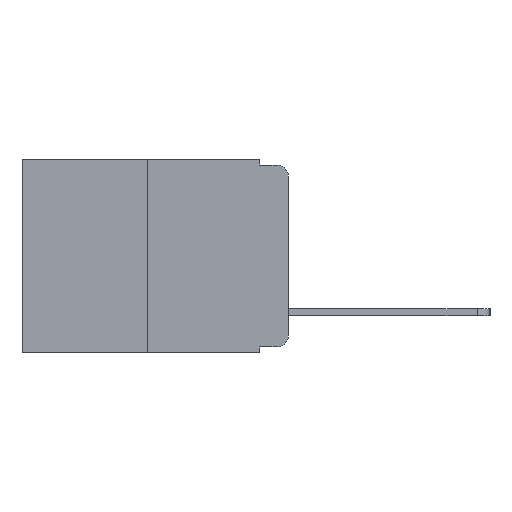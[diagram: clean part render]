
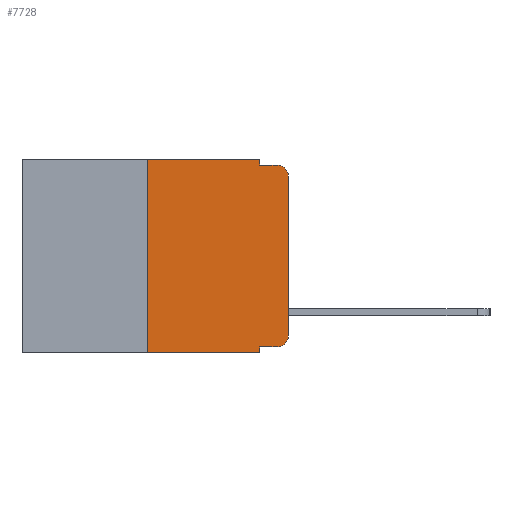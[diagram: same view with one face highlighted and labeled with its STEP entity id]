
A CAD part, left-side view. The second image highlights one B-rep face of the part: STEP entity #7728.
In plain terms, the highlighted planar face has unit normal (-1, 0, 0).
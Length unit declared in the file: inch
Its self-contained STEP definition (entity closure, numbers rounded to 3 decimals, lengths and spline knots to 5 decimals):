
#98 = DIRECTION ( 'NONE',  ( 0., -1., 0. ) ) ;
#183 = DIRECTION ( 'NONE',  ( 0., 0., -1. ) ) ;
#267 = ORIENTED_EDGE ( 'NONE', *, *, #5703, .T. ) ;
#307 = EDGE_CURVE ( 'NONE', #10371, #6859, #8863, .T. ) ;
#336 = CARTESIAN_POINT ( 'NONE',  ( 0., 0.473, 0. ) ) ;
#429 = LINE ( 'NONE', #5321, #7722 ) ;
#597 = ORIENTED_EDGE ( 'NONE', *, *, #5041, .T. ) ;
#945 = ORIENTED_EDGE ( 'NONE', *, *, #9875, .T. ) ;
#980 = ORIENTED_EDGE ( 'NONE', *, *, #4380, .F. ) ;
#998 = EDGE_CURVE ( 'NONE', #8926, #10371, #9156, .T. ) ;
#1080 = ORIENTED_EDGE ( 'NONE', *, *, #10041, .F. ) ;
#1398 = DIRECTION ( 'NONE',  ( 0., 0., -1. ) ) ;
#1710 = VECTOR ( 'NONE', #2047, 39.37008 ) ;
#1717 = EDGE_CURVE ( 'NONE', #8926, #1913, #6470, .T. ) ;
#1743 = ORIENTED_EDGE ( 'NONE', *, *, #307, .T. ) ;
#1839 = LINE ( 'NONE', #11655, #6770 ) ;
#1913 = VERTEX_POINT ( 'NONE', #4259 ) ;
#2047 = DIRECTION ( 'NONE',  ( 0., -1., 0. ) ) ;
#2114 = ORIENTED_EDGE ( 'NONE', *, *, #2402, .F. ) ;
#2126 = ORIENTED_EDGE ( 'NONE', *, *, #998, .T. ) ;
#2197 = CARTESIAN_POINT ( 'NONE',  ( 0., 0.473, 0. ) ) ;
#2402 = EDGE_CURVE ( 'NONE', #5201, #11001, #6900, .T. ) ;
#2627 = ORIENTED_EDGE ( 'NONE', *, *, #3727, .F. ) ;
#2981 = VECTOR ( 'NONE', #3677, 39.37008 ) ;
#3305 = LINE ( 'NONE', #3436, #2981 ) ;
#3384 = PLANE ( 'NONE',  #4681 ) ;
#3436 = CARTESIAN_POINT ( 'NONE',  ( 0., 0.051, -0.01 ) ) ;
#3589 = ORIENTED_EDGE ( 'NONE', *, *, #1717, .F. ) ;
#3677 = DIRECTION ( 'NONE',  ( 0., -1., 0. ) ) ;
#3727 = EDGE_CURVE ( 'NONE', #11915, #7376, #429, .T. ) ;
#3872 = VERTEX_POINT ( 'NONE', #8337 ) ;
#3969 = EDGE_LOOP ( 'NONE', ( #267, #597, #980, #2627, #1080, #2114, #945, #3589, #2126, #1743 ) ) ;
#3997 = CARTESIAN_POINT ( 'NONE',  ( 0., 0., -0.313 ) ) ;
#4040 = CARTESIAN_POINT ( 'NONE',  ( 0., 0.051, 0. ) ) ;
#4085 = CARTESIAN_POINT ( 'NONE',  ( 0., 0.02, -0.03 ) ) ;
#4259 = CARTESIAN_POINT ( 'NONE',  ( 0., 0.051, -0.343 ) ) ;
#4288 = CARTESIAN_POINT ( 'NONE',  ( 0., 0.25, -0.343 ) ) ;
#4380 = EDGE_CURVE ( 'NONE', #7376, #3872, #3305, .T. ) ;
#4681 = AXIS2_PLACEMENT_3D ( 'NONE', #336, #7291, #1398 ) ;
#5041 = EDGE_CURVE ( 'NONE', #6002, #3872, #6338, .T. ) ;
#5081 = DIRECTION ( 'NONE',  ( 0., 0., -1. ) ) ;
#5201 = VERTEX_POINT ( 'NONE', #4288 ) ;
#5319 = DIRECTION ( 'NONE',  ( 0., 0., -1. ) ) ;
#5321 = CARTESIAN_POINT ( 'NONE',  ( 0., 0.051, 0. ) ) ;
#5378 = FACE_OUTER_BOUND ( 'NONE', #3969, .T. ) ;
#5703 = EDGE_CURVE ( 'NONE', #6859, #6002, #1839, .T. ) ;
#5932 = CARTESIAN_POINT ( 'NONE',  ( 0., 0.02, -0.313 ) ) ;
#5958 = DIRECTION ( 'NONE',  ( -1., 0., 0. ) ) ;
#6002 = VERTEX_POINT ( 'NONE', #11251 ) ;
#6338 = CIRCLE ( 'NONE', #10203, 0.02 ) ;
#6470 = LINE ( 'NONE', #4040, #11123 ) ;
#6675 = CARTESIAN_POINT ( 'NONE',  ( 0., 0.051, -0.01 ) ) ;
#6770 = VECTOR ( 'NONE', #8041, 39.37008 ) ;
#6859 = VERTEX_POINT ( 'NONE', #3997 ) ;
#6900 = LINE ( 'NONE', #11767, #11255 ) ;
#7034 = VECTOR ( 'NONE', #11322, 39.37008 ) ;
#7291 = DIRECTION ( 'NONE',  ( 1., 0., 0. ) ) ;
#7376 = VERTEX_POINT ( 'NONE', #6675 ) ;
#7722 = VECTOR ( 'NONE', #11535, 39.37008 ) ;
#7728 = ADVANCED_FACE ( 'NONE', ( #5378 ), #3384, .F. ) ;
#7773 = VECTOR ( 'NONE', #98, 39.37008 ) ;
#7925 = LINE ( 'NONE', #12233, #7034 ) ;
#8041 = DIRECTION ( 'NONE',  ( 0., 0., 1. ) ) ;
#8098 = CARTESIAN_POINT ( 'NONE',  ( 0., 0.051, 0. ) ) ;
#8135 = CARTESIAN_POINT ( 'NONE',  ( 0., 0.051, -0.333 ) ) ;
#8337 = CARTESIAN_POINT ( 'NONE',  ( 0., 0.02, -0.01 ) ) ;
#8863 = CIRCLE ( 'NONE', #10957, 0.02 ) ;
#8926 = VERTEX_POINT ( 'NONE', #8135 ) ;
#9156 = LINE ( 'NONE', #9550, #1710 ) ;
#9550 = CARTESIAN_POINT ( 'NONE',  ( 0., 0.051, -0.333 ) ) ;
#9875 = EDGE_CURVE ( 'NONE', #5201, #1913, #7925, .T. ) ;
#9987 = DIRECTION ( 'NONE',  ( 0., 0., 1. ) ) ;
#10041 = EDGE_CURVE ( 'NONE', #11001, #11915, #10518, .T. ) ;
#10203 = AXIS2_PLACEMENT_3D ( 'NONE', #4085, #10714, #5081 ) ;
#10371 = VERTEX_POINT ( 'NONE', #11199 ) ;
#10492 = CARTESIAN_POINT ( 'NONE',  ( 0., 0.25, 0. ) ) ;
#10518 = LINE ( 'NONE', #2197, #7773 ) ;
#10714 = DIRECTION ( 'NONE',  ( -1., 0., 0. ) ) ;
#10957 = AXIS2_PLACEMENT_3D ( 'NONE', #5932, #5958, #5319 ) ;
#11001 = VERTEX_POINT ( 'NONE', #10492 ) ;
#11123 = VECTOR ( 'NONE', #183, 39.37008 ) ;
#11199 = CARTESIAN_POINT ( 'NONE',  ( 0., 0.02, -0.333 ) ) ;
#11251 = CARTESIAN_POINT ( 'NONE',  ( 0., 0., -0.03 ) ) ;
#11255 = VECTOR ( 'NONE', #9987, 39.37008 ) ;
#11322 = DIRECTION ( 'NONE',  ( 0., -1., 0. ) ) ;
#11535 = DIRECTION ( 'NONE',  ( 0., 0., -1. ) ) ;
#11655 = CARTESIAN_POINT ( 'NONE',  ( 0., 0., 0. ) ) ;
#11767 = CARTESIAN_POINT ( 'NONE',  ( 0., 0.25, 0. ) ) ;
#11915 = VERTEX_POINT ( 'NONE', #8098 ) ;
#12233 = CARTESIAN_POINT ( 'NONE',  ( 0., 0.473, -0.343 ) ) ;
